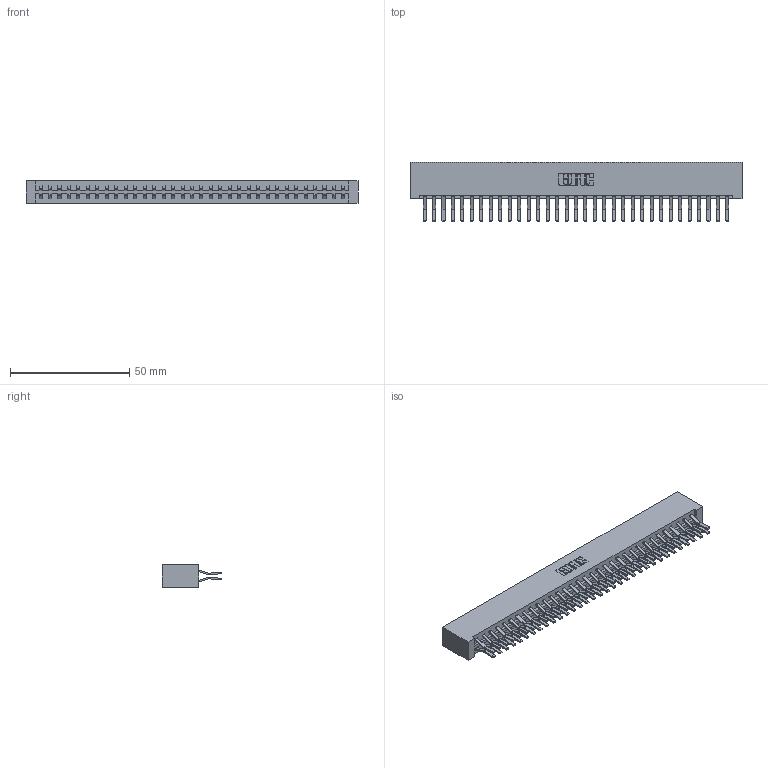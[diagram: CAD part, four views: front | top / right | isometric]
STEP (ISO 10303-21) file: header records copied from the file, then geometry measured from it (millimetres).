
FILE_DESCRIPTION (( 'STEP AP203' ), '1' );
FILE_NAME ('833-066-560-201.STEP', '2020-06-05T09:47:51', ( '' ), ( '' ), 'SwSTEP 2.0', 'SolidWorks 2020', '' );
FILE_SCHEMA (( 'CONFIG_CONTROL_DESIGN' ));
Length unit declared in the file: inch
Products named in the file (3): 345-292-001_560 Tail; 833-066-560-201; 833 Part_Lugless
Assembly tree (67 placements, depth 2):
  833-066-560-201
    833 Part_Lugless
    345-292-001_560 Tail  x66
Bounding box: 139.01 x 24.78 x 9.4 mm (x, y, z)
Volume: 15173.2 mm3; surface area: 19100.2 mm2
Topology: 67 solids, 67 shells, 3670 faces, 10913 edges, 7186 vertices
Faces by surface type: plane 2442, cylinder 1228
Entity records: 22205 total; most frequent: CARTESIAN_POINT 3690, ORIENTED_EDGE 3626, DIRECTION 3165, EDGE_CURVE 1813, LINE 1689, VECTOR 1689, VERTEX_POINT 1206, AXIS2_PLACEMENT_3D 738
